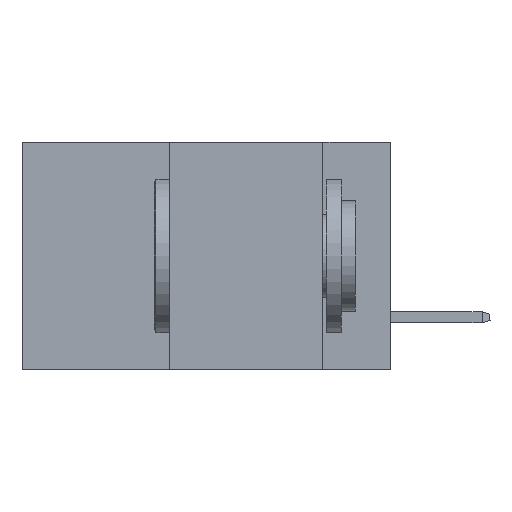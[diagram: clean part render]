
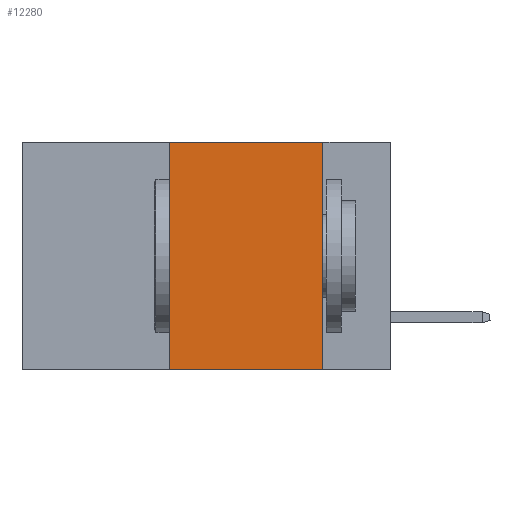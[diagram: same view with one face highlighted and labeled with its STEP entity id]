
A CAD part, left-side view. The second image highlights one B-rep face of the part: STEP entity #12280.
In plain terms, the highlighted planar face has unit normal (-1, 0, 0).
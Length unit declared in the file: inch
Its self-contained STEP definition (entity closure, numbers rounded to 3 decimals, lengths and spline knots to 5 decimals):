
#1434 = ORIENTED_EDGE ( 'NONE', *, *, #18726, .F. ) ;
#2418 = CARTESIAN_POINT ( 'NONE',  ( 0., 0.36, 0. ) ) ;
#2608 = VECTOR ( 'NONE', #3586, 39.37008 ) ;
#2653 = DIRECTION ( 'NONE',  ( 1., 0., 0. ) ) ;
#3096 = CARTESIAN_POINT ( 'NONE',  ( 0., 0.6, -0.37 ) ) ;
#3137 = LINE ( 'NONE', #6800, #2608 ) ;
#3586 = DIRECTION ( 'NONE',  ( 0., -1., 0. ) ) ;
#4202 = PLANE ( 'NONE',  #7644 ) ;
#5440 = CARTESIAN_POINT ( 'NONE',  ( 0., 0.11, 0. ) ) ;
#6520 = EDGE_CURVE ( 'NONE', #12553, #21259, #11261, .T. ) ;
#6800 = CARTESIAN_POINT ( 'NONE',  ( 0., 0.6, 0. ) ) ;
#6873 = VECTOR ( 'NONE', #11398, 39.37008 ) ;
#7099 = ORIENTED_EDGE ( 'NONE', *, *, #14742, .F. ) ;
#7409 = LINE ( 'NONE', #3096, #6873 ) ;
#7644 = AXIS2_PLACEMENT_3D ( 'NONE', #12804, #2653, #21278 ) ;
#9985 = EDGE_LOOP ( 'NONE', ( #14306, #7099, #1434, #12058 ) ) ;
#11261 = LINE ( 'NONE', #5440, #19204 ) ;
#11398 = DIRECTION ( 'NONE',  ( 0., -1., 0. ) ) ;
#11422 = CARTESIAN_POINT ( 'NONE',  ( 0., 0.11, -0.37 ) ) ;
#11537 = CARTESIAN_POINT ( 'NONE',  ( 0., 0.11, 0. ) ) ;
#12058 = ORIENTED_EDGE ( 'NONE', *, *, #21947, .T. ) ;
#12280 = ADVANCED_FACE ( 'NONE', ( #20467 ), #4202, .F. ) ;
#12553 = VERTEX_POINT ( 'NONE', #11537 ) ;
#12564 = VECTOR ( 'NONE', #14957, 39.37008 ) ;
#12804 = CARTESIAN_POINT ( 'NONE',  ( 0., 0.6, 0. ) ) ;
#13538 = CARTESIAN_POINT ( 'NONE',  ( 0., 0.36, 0. ) ) ;
#14306 = ORIENTED_EDGE ( 'NONE', *, *, #6520, .F. ) ;
#14742 = EDGE_CURVE ( 'NONE', #20144, #12553, #3137, .T. ) ;
#14957 = DIRECTION ( 'NONE',  ( 0., 0., 1. ) ) ;
#16999 = VERTEX_POINT ( 'NONE', #20051 ) ;
#17059 = LINE ( 'NONE', #2418, #12564 ) ;
#17506 = DIRECTION ( 'NONE',  ( 0., 0., -1. ) ) ;
#18726 = EDGE_CURVE ( 'NONE', #16999, #20144, #17059, .T. ) ;
#19204 = VECTOR ( 'NONE', #17506, 39.37008 ) ;
#20051 = CARTESIAN_POINT ( 'NONE',  ( 0., 0.36, -0.37 ) ) ;
#20144 = VERTEX_POINT ( 'NONE', #13538 ) ;
#20467 = FACE_OUTER_BOUND ( 'NONE', #9985, .T. ) ;
#21259 = VERTEX_POINT ( 'NONE', #11422 ) ;
#21278 = DIRECTION ( 'NONE',  ( 0., 0., -1. ) ) ;
#21947 = EDGE_CURVE ( 'NONE', #16999, #21259, #7409, .T. ) ;
